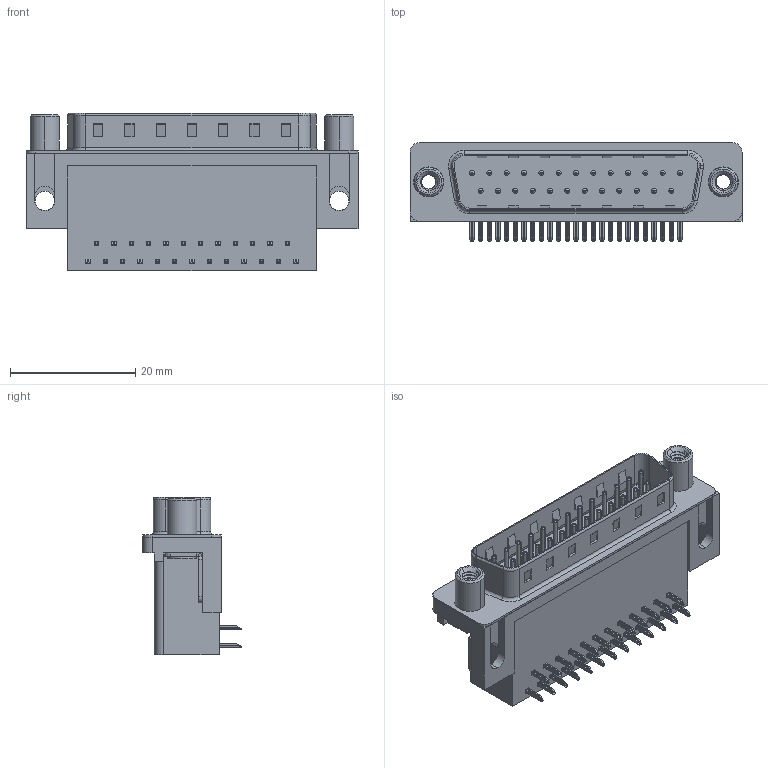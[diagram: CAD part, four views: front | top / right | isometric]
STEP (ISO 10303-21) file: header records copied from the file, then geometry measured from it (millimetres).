
FILE_DESCRIPTION (( 'STEP AP203' ), '1' );
FILE_NAME ('625-025-662-510.STEP', '2018-11-06T03:41:29', ( '' ), ( '' ), 'SwSTEP 2.0', 'SolidWorks 2016', '' );
FILE_SCHEMA (( 'CONFIG_CONTROL_DESIGN' ));
Length unit declared in the file: millimetre
Products named in the file (7): 625-025-662-510; 625 Housing_25 Socket; 625 Shell_25 Socket; 625 Contact Bottom; 625 Contact Top; 625 Thru Hole Board Mount; 625 Round Threaded Standoff
Assembly tree (31 placements, depth 2):
  625-025-662-510
    625 Housing_25 Socket
    625 Shell_25 Socket
    625 Contact Bottom  x12
    625 Contact Top  x13
    625 Thru Hole Board Mount  x2
    625 Round Threaded Standoff  x2
Bounding box: 53.04 x 15.73 x 25.16 mm (x, y, z)
Volume: 9252.3 mm3; surface area: 9047.9 mm2
Topology: 31 solids, 31 shells, 2259 faces, 5613 edges, 3471 vertices
Faces by surface type: plane 1397, cylinder 669, torus 165, bspline 16, cone 12
Entity records: 22807 total; most frequent: CARTESIAN_POINT 5351, DIRECTION 3360, ORIENTED_EDGE 3276, EDGE_CURVE 1638, LINE 1148, VECTOR 1148, AXIS2_PLACEMENT_3D 1106, VERTEX_POINT 1053
